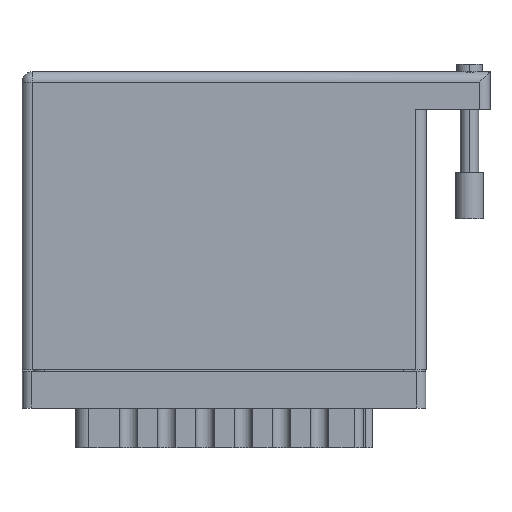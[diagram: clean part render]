
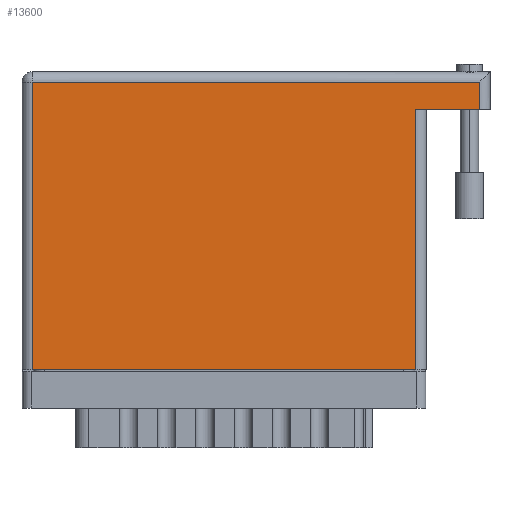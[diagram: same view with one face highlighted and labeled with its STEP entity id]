
A CAD part, front view. The second image highlights one B-rep face of the part: STEP entity #13600.
In plain terms, the highlighted face is planar.
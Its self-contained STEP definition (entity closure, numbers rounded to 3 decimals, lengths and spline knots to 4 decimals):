
#2337 = CARTESIAN_POINT ( 'NONE',  ( 0.07, 0., 0. ) ) ;
#3737 = LINE ( 'NONE', #11176, #72343 ) ;
#3765 = CARTESIAN_POINT ( 'NONE',  ( 3.12, 2.03, 0. ) ) ;
#5033 = DIRECTION ( 'NONE',  ( -1., 0., 0. ) ) ;
#5053 = VECTOR ( 'NONE', #51633, 39.3701 ) ;
#9363 = EDGE_LOOP ( 'NONE', ( #11266, #67411, #63883, #23038, #37541, #37255 ) ) ;
#9680 = EDGE_CURVE ( 'NONE', #40281, #43793, #49791, .T. ) ;
#10334 = VERTEX_POINT ( 'NONE', #78853 ) ;
#11176 = CARTESIAN_POINT ( 'NONE',  ( 0., 0., 0. ) ) ;
#11266 = ORIENTED_EDGE ( 'NONE', *, *, #75499, .T. ) ;
#13600 = ADVANCED_FACE ( 'NONE', ( #53266 ), #46036, .F. ) ;
#13907 = CARTESIAN_POINT ( 'NONE',  ( 2.685, 1.774, 0. ) ) ;
#17037 = LINE ( 'NONE', #3765, #34649 ) ;
#23038 = ORIENTED_EDGE ( 'NONE', *, *, #68024, .T. ) ;
#23991 = CARTESIAN_POINT ( 'NONE',  ( 0., 1.96, 0. ) ) ;
#28538 = LINE ( 'NONE', #23991, #67991 ) ;
#31841 = DIRECTION ( 'NONE',  ( 0., 0., -1. ) ) ;
#33387 = DIRECTION ( 'NONE',  ( 0., 1., 0. ) ) ;
#34194 = VECTOR ( 'NONE', #48889, 39.3701 ) ;
#34649 = VECTOR ( 'NONE', #50280, 39.3701 ) ;
#37255 = ORIENTED_EDGE ( 'NONE', *, *, #56699, .T. ) ;
#37541 = ORIENTED_EDGE ( 'NONE', *, *, #44718, .T. ) ;
#40281 = VERTEX_POINT ( 'NONE', #80179 ) ;
#43793 = VERTEX_POINT ( 'NONE', #73753 ) ;
#43992 = VERTEX_POINT ( 'NONE', #83694 ) ;
#44381 = CARTESIAN_POINT ( 'NONE',  ( 3.12, 1.96, 0. ) ) ;
#44718 = EDGE_CURVE ( 'NONE', #83917, #56216, #28538, .T. ) ;
#45283 = CARTESIAN_POINT ( 'NONE',  ( 3.19, 1.774, 0. ) ) ;
#46036 = PLANE ( 'NONE',  #46264 ) ;
#46264 = AXIS2_PLACEMENT_3D ( 'NONE', #65174, #31841, #5033 ) ;
#48889 = DIRECTION ( 'NONE',  ( 0., -1., 0. ) ) ;
#49454 = VECTOR ( 'NONE', #33387, 39.3701 ) ;
#49791 = LINE ( 'NONE', #45283, #5053 ) ;
#50280 = DIRECTION ( 'NONE',  ( 0., 1., 0. ) ) ;
#51165 = EDGE_CURVE ( 'NONE', #10334, #43793, #84872, .T. ) ;
#51633 = DIRECTION ( 'NONE',  ( -1., 0., 0. ) ) ;
#53266 = FACE_OUTER_BOUND ( 'NONE', #9363, .T. ) ;
#56216 = VERTEX_POINT ( 'NONE', #76571 ) ;
#56699 = EDGE_CURVE ( 'NONE', #56216, #43992, #70458, .T. ) ;
#63883 = ORIENTED_EDGE ( 'NONE', *, *, #9680, .F. ) ;
#65174 = CARTESIAN_POINT ( 'NONE',  ( 0., 2.03, 0. ) ) ;
#67411 = ORIENTED_EDGE ( 'NONE', *, *, #51165, .T. ) ;
#67991 = VECTOR ( 'NONE', #77115, 39.3701 ) ;
#68024 = EDGE_CURVE ( 'NONE', #40281, #83917, #17037, .T. ) ;
#70458 = LINE ( 'NONE', #2337, #34194 ) ;
#70684 = DIRECTION ( 'NONE',  ( 1., 0., 0. ) ) ;
#72343 = VECTOR ( 'NONE', #70684, 39.3701 ) ;
#73753 = CARTESIAN_POINT ( 'NONE',  ( 2.685, 1.774, 0. ) ) ;
#75499 = EDGE_CURVE ( 'NONE', #43992, #10334, #3737, .T. ) ;
#76571 = CARTESIAN_POINT ( 'NONE',  ( 0.07, 1.96, 0. ) ) ;
#77115 = DIRECTION ( 'NONE',  ( -1., 0., 0. ) ) ;
#78853 = CARTESIAN_POINT ( 'NONE',  ( 2.685, 0., 0. ) ) ;
#80179 = CARTESIAN_POINT ( 'NONE',  ( 3.12, 1.774, 0. ) ) ;
#83694 = CARTESIAN_POINT ( 'NONE',  ( 0.07, 0., 0. ) ) ;
#83917 = VERTEX_POINT ( 'NONE', #44381 ) ;
#84872 = LINE ( 'NONE', #13907, #49454 ) ;
